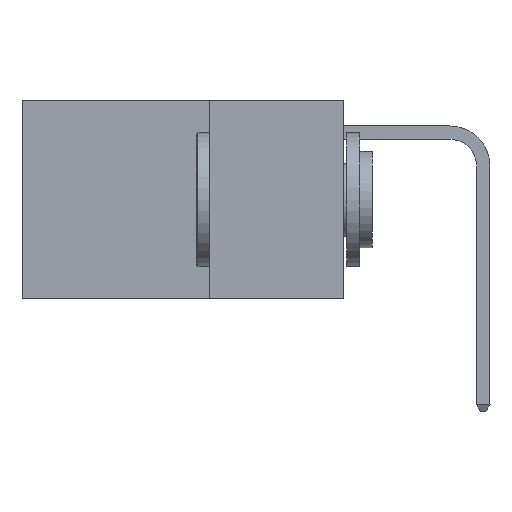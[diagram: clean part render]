
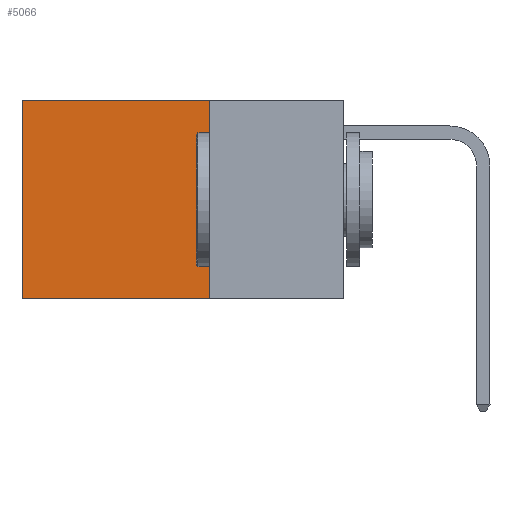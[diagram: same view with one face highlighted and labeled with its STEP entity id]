
A CAD part, left-side view. The second image highlights one B-rep face of the part: STEP entity #5066.
In plain terms, the highlighted planar face has unit normal (-1, 0, 0).
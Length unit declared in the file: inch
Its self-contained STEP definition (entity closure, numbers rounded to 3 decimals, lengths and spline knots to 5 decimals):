
#302 = EDGE_CURVE ( 'NONE', #5421, #12147, #935, .T. ) ;
#791 = CARTESIAN_POINT ( 'NONE',  ( 0.2625, 0.25, 0. ) ) ;
#935 = LINE ( 'NONE', #3114, #11261 ) ;
#1633 = VECTOR ( 'NONE', #11957, 39.37008 ) ;
#1782 = CARTESIAN_POINT ( 'NONE',  ( 0.2625, 0.25, 0. ) ) ;
#1978 = CARTESIAN_POINT ( 'NONE',  ( 0.2625, 0.25, 0. ) ) ;
#2619 = EDGE_LOOP ( 'NONE', ( #10695, #7234, #8757, #9241 ) ) ;
#3114 = CARTESIAN_POINT ( 'NONE',  ( 0.2625, 0.25, 0. ) ) ;
#3668 = LINE ( 'NONE', #9606, #5472 ) ;
#3976 = LINE ( 'NONE', #1978, #1633 ) ;
#4177 = EDGE_CURVE ( 'NONE', #8927, #7905, #3668, .T. ) ;
#4757 = DIRECTION ( 'NONE',  ( 0., 1., 0. ) ) ;
#5066 = ADVANCED_FACE ( 'NONE', ( #6458 ), #12466, .F. ) ;
#5412 = AXIS2_PLACEMENT_3D ( 'NONE', #1782, #5685, #9582 ) ;
#5421 = VERTEX_POINT ( 'NONE', #791 ) ;
#5472 = VECTOR ( 'NONE', #4757, 39.37008 ) ;
#5552 = CARTESIAN_POINT ( 'NONE',  ( 0.2625, 0.25, -0.37 ) ) ;
#5685 = DIRECTION ( 'NONE',  ( 1., 0., 0. ) ) ;
#5953 = VECTOR ( 'NONE', #9357, 39.37008 ) ;
#6458 = FACE_OUTER_BOUND ( 'NONE', #2619, .T. ) ;
#6546 = CARTESIAN_POINT ( 'NONE',  ( 0.2625, 0.6, 0. ) ) ;
#7234 = ORIENTED_EDGE ( 'NONE', *, *, #4177, .F. ) ;
#7554 = CARTESIAN_POINT ( 'NONE',  ( 0.2625, 0.6, 0. ) ) ;
#7905 = VERTEX_POINT ( 'NONE', #12246 ) ;
#8648 = EDGE_CURVE ( 'NONE', #5421, #8927, #3976, .T. ) ;
#8757 = ORIENTED_EDGE ( 'NONE', *, *, #8648, .F. ) ;
#8927 = VERTEX_POINT ( 'NONE', #5552 ) ;
#9241 = ORIENTED_EDGE ( 'NONE', *, *, #302, .T. ) ;
#9357 = DIRECTION ( 'NONE',  ( 0., 0., -1. ) ) ;
#9582 = DIRECTION ( 'NONE',  ( 0., 0., -1. ) ) ;
#9606 = CARTESIAN_POINT ( 'NONE',  ( 0.2625, 0.25, -0.37 ) ) ;
#10695 = ORIENTED_EDGE ( 'NONE', *, *, #12081, .T. ) ;
#11261 = VECTOR ( 'NONE', #11924, 39.37008 ) ;
#11476 = LINE ( 'NONE', #7554, #5953 ) ;
#11924 = DIRECTION ( 'NONE',  ( 0., 1., 0. ) ) ;
#11957 = DIRECTION ( 'NONE',  ( 0., 0., -1. ) ) ;
#12081 = EDGE_CURVE ( 'NONE', #12147, #7905, #11476, .T. ) ;
#12147 = VERTEX_POINT ( 'NONE', #6546 ) ;
#12246 = CARTESIAN_POINT ( 'NONE',  ( 0.2625, 0.6, -0.37 ) ) ;
#12466 = PLANE ( 'NONE',  #5412 ) ;
